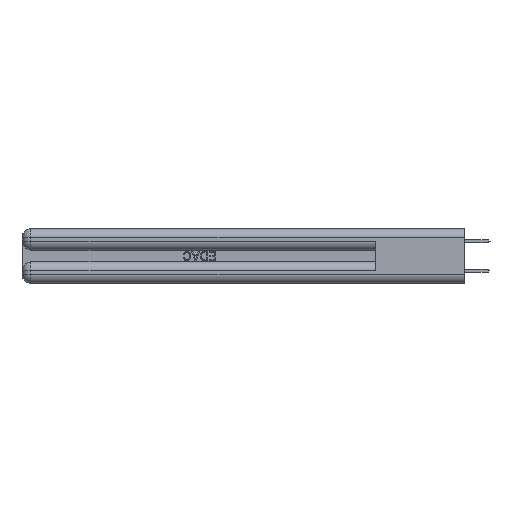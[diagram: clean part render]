
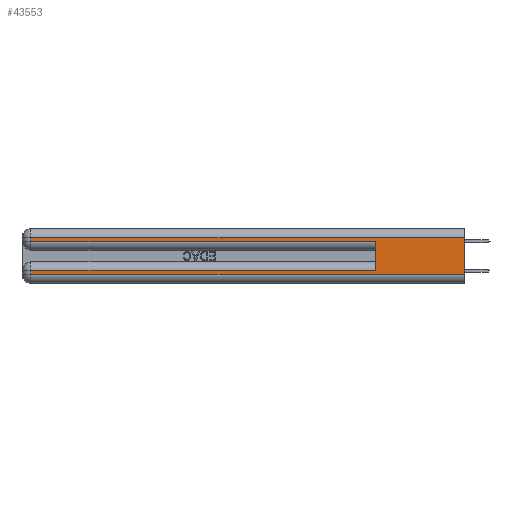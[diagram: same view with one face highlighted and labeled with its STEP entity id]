
A CAD part, left-side view. The second image highlights one B-rep face of the part: STEP entity #43553.
In plain terms, the highlighted planar face has unit normal (-1, 0, 0).
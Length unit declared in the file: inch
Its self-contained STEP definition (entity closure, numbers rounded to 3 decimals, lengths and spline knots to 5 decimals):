
#1375 = EDGE_LOOP ( 'NONE', ( #27658, #14903, #27789, #6217, #32959, #42184, #41030, #45183 ) ) ;
#4551 = DIRECTION ( 'NONE',  ( 0., -1., 0. ) ) ;
#5364 = LINE ( 'NONE', #16944, #6972 ) ;
#6108 = EDGE_CURVE ( 'NONE', #29254, #38112, #27795, .T. ) ;
#6217 = ORIENTED_EDGE ( 'NONE', *, *, #33557, .T. ) ;
#6890 = EDGE_CURVE ( 'NONE', #35322, #12632, #13975, .T. ) ;
#6972 = VECTOR ( 'NONE', #21007, 39.37008 ) ;
#7648 = DIRECTION ( 'NONE',  ( 0., 0., -1. ) ) ;
#8691 = DIRECTION ( 'NONE',  ( 0., -1., 0. ) ) ;
#9061 = VECTOR ( 'NONE', #11262, 39.37008 ) ;
#9159 = CARTESIAN_POINT ( 'NONE',  ( 0., 0., 0.06 ) ) ;
#9291 = VECTOR ( 'NONE', #8691, 39.37008 ) ;
#10355 = CARTESIAN_POINT ( 'NONE',  ( 0., 0., 0.31 ) ) ;
#11262 = DIRECTION ( 'NONE',  ( 0., 0., 1. ) ) ;
#11542 = LINE ( 'NONE', #41126, #24208 ) ;
#12502 = DIRECTION ( 'NONE',  ( 0., 1., 0. ) ) ;
#12632 = VERTEX_POINT ( 'NONE', #29482 ) ;
#13975 = LINE ( 'NONE', #41143, #9061 ) ;
#14903 = ORIENTED_EDGE ( 'NONE', *, *, #6108, .T. ) ;
#15429 = CARTESIAN_POINT ( 'NONE',  ( 0., 2.94, 0.06 ) ) ;
#15848 = EDGE_CURVE ( 'NONE', #19709, #37050, #16668, .T. ) ;
#16255 = EDGE_CURVE ( 'NONE', #29254, #42282, #23705, .T. ) ;
#16358 = CARTESIAN_POINT ( 'NONE',  ( 0., 0., 0.37 ) ) ;
#16656 = PLANE ( 'NONE',  #32542 ) ;
#16668 = LINE ( 'NONE', #25455, #42490 ) ;
#16944 = CARTESIAN_POINT ( 'NONE',  ( 0., 2.94, 0.37 ) ) ;
#17537 = LINE ( 'NONE', #9159, #9291 ) ;
#19709 = VERTEX_POINT ( 'NONE', #23413 ) ;
#21007 = DIRECTION ( 'NONE',  ( 0., 0., -1. ) ) ;
#21980 = FACE_OUTER_BOUND ( 'NONE', #1375, .T. ) ;
#22003 = CARTESIAN_POINT ( 'NONE',  ( 0., 0., 0.285 ) ) ;
#23225 = CARTESIAN_POINT ( 'NONE',  ( 0., 2.94, 0.285 ) ) ;
#23413 = CARTESIAN_POINT ( 'NONE',  ( 0., 2.94, 0.085 ) ) ;
#23705 = LINE ( 'NONE', #26760, #39675 ) ;
#24208 = VECTOR ( 'NONE', #12502, 39.37008 ) ;
#24648 = CARTESIAN_POINT ( 'NONE',  ( 0., 2.94, 0.31 ) ) ;
#25455 = CARTESIAN_POINT ( 'NONE',  ( 0., 2.94, 0.37 ) ) ;
#26760 = CARTESIAN_POINT ( 'NONE',  ( 0., 0., 0.37 ) ) ;
#27658 = ORIENTED_EDGE ( 'NONE', *, *, #16255, .F. ) ;
#27789 = ORIENTED_EDGE ( 'NONE', *, *, #41789, .T. ) ;
#27795 = LINE ( 'NONE', #10355, #39335 ) ;
#28025 = VECTOR ( 'NONE', #4551, 39.37008 ) ;
#29254 = VERTEX_POINT ( 'NONE', #30449 ) ;
#29482 = CARTESIAN_POINT ( 'NONE',  ( 0., 0.6, 0.285 ) ) ;
#30449 = CARTESIAN_POINT ( 'NONE',  ( 0., 0., 0.31 ) ) ;
#31982 = DIRECTION ( 'NONE',  ( 0., 1., 0. ) ) ;
#32542 = AXIS2_PLACEMENT_3D ( 'NONE', #16358, #40665, #40969 ) ;
#32844 = EDGE_CURVE ( 'NONE', #35322, #19709, #11542, .T. ) ;
#32959 = ORIENTED_EDGE ( 'NONE', *, *, #6890, .F. ) ;
#33557 = EDGE_CURVE ( 'NONE', #35875, #12632, #34067, .T. ) ;
#33726 = EDGE_CURVE ( 'NONE', #37050, #42282, #17537, .T. ) ;
#33803 = DIRECTION ( 'NONE',  ( 0., 0., -1. ) ) ;
#34067 = LINE ( 'NONE', #22003, #28025 ) ;
#34332 = CARTESIAN_POINT ( 'NONE',  ( 0., 0.6, 0.085 ) ) ;
#35322 = VERTEX_POINT ( 'NONE', #34332 ) ;
#35875 = VERTEX_POINT ( 'NONE', #23225 ) ;
#37050 = VERTEX_POINT ( 'NONE', #15429 ) ;
#38112 = VERTEX_POINT ( 'NONE', #24648 ) ;
#39335 = VECTOR ( 'NONE', #31982, 39.37008 ) ;
#39675 = VECTOR ( 'NONE', #33803, 39.37008 ) ;
#40665 = DIRECTION ( 'NONE',  ( 1., 0., 0. ) ) ;
#40912 = CARTESIAN_POINT ( 'NONE',  ( 0., 0., 0.06 ) ) ;
#40969 = DIRECTION ( 'NONE',  ( 0., 0., -1. ) ) ;
#41030 = ORIENTED_EDGE ( 'NONE', *, *, #15848, .T. ) ;
#41126 = CARTESIAN_POINT ( 'NONE',  ( 0., 0., 0.085 ) ) ;
#41143 = CARTESIAN_POINT ( 'NONE',  ( 0., 0.6, 0.145 ) ) ;
#41789 = EDGE_CURVE ( 'NONE', #38112, #35875, #5364, .T. ) ;
#42184 = ORIENTED_EDGE ( 'NONE', *, *, #32844, .T. ) ;
#42282 = VERTEX_POINT ( 'NONE', #40912 ) ;
#42490 = VECTOR ( 'NONE', #7648, 39.37008 ) ;
#43553 = ADVANCED_FACE ( 'NONE', ( #21980 ), #16656, .F. ) ;
#45183 = ORIENTED_EDGE ( 'NONE', *, *, #33726, .T. ) ;
